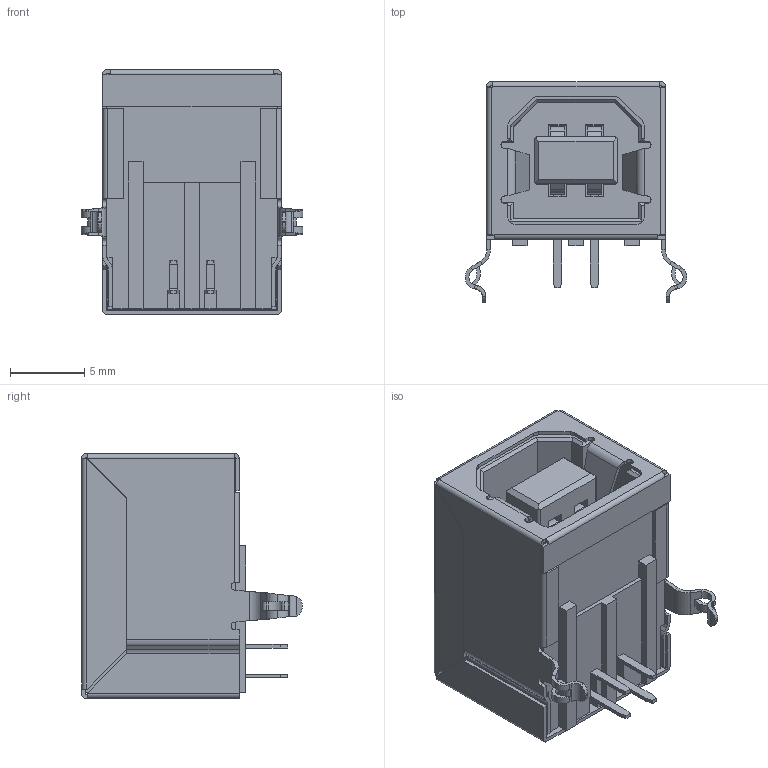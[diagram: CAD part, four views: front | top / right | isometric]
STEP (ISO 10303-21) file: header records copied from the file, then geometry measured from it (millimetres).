
FILE_DESCRIPTION (( 'STEP AP214' ), '1' );
FILE_NAME ('690P204-123-211.STEP', '2021-01-14T20:14:49', ( '' ), ( '' ), 'SwSTEP 2.0', 'SolidWorks 2020', '' );
FILE_SCHEMA (( 'AUTOMOTIVE_DESIGN' ));
Length unit declared in the file: millimetre
Products named in the file (5): SHELL 690P204-X23-2XX; CONTACT 690P204-X23-2XX; INSULATOR 690P204-X23-2XX_Black; CONTACT01 690P204-X23-2XX; 690P204-123-211
Assembly tree (6 placements, depth 2):
  690P204-123-211
    SHELL 690P204-X23-2XX
    INSULATOR 690P204-X23-2XX_Black
    CONTACT 690P204-X23-2XX  x2
    CONTACT01 690P204-X23-2XX  x2
Bounding box: 14.94 x 14.87 x 16.5 mm (x, y, z)
Volume: 1498.8 mm3; surface area: 3520.8 mm2
Topology: 6 solids, 6 shells, 631 faces, 1757 edges, 1124 vertices
Faces by surface type: plane 436, cylinder 167, bspline 28
Entity records: 16982 total; most frequent: CARTESIAN_POINT 3885, ORIENTED_EDGE 2800, DIRECTION 2550, EDGE_CURVE 1400, LINE 1112, VECTOR 1112, VERTEX_POINT 886, AXIS2_PLACEMENT_3D 719
